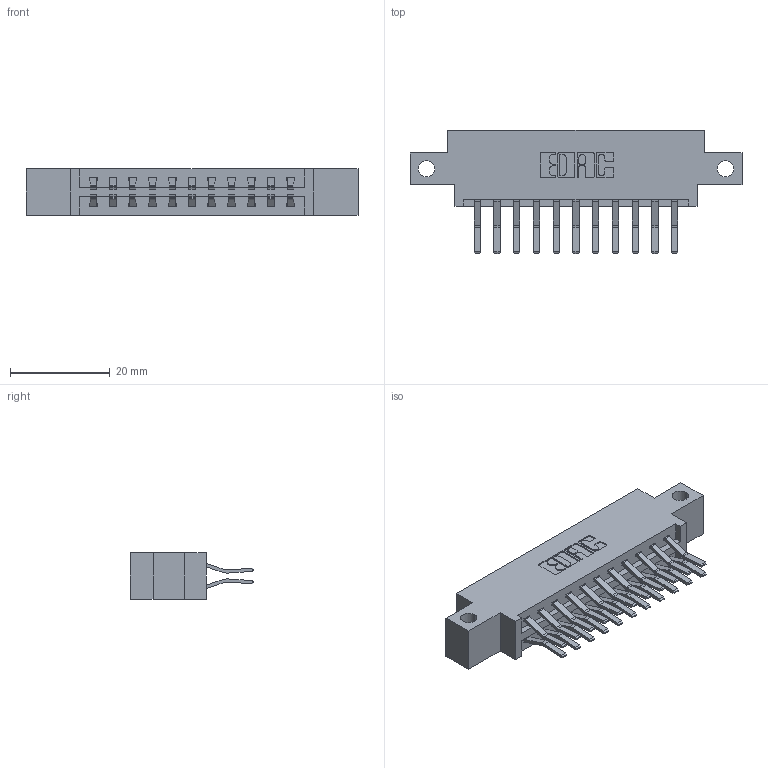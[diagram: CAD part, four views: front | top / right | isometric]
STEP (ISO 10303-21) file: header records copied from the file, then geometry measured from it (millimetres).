
FILE_DESCRIPTION (( 'STEP AP203' ), '1' );
FILE_NAME ('337-022-560-812.STEP', '2018-08-05T16:03:02', ( '' ), ( '' ), 'SwSTEP 2.0', 'SolidWorks 2016', '' );
FILE_SCHEMA (( 'CONFIG_CONTROL_DESIGN' ));
Length unit declared in the file: inch
Products named in the file (3): 337 Part_0.170 Offset - Side Mount; 345-292-001_560 Tail; 337-022-560-812
Assembly tree (23 placements, depth 2):
  337-022-560-812
    337 Part_0.170 Offset - Side Mount
    345-292-001_560 Tail  x22
Bounding box: 66.6 x 24.78 x 9.4 mm (x, y, z)
Volume: 6545.5 mm3; surface area: 7470.5 mm2
Topology: 23 solids, 23 shells, 1350 faces, 3997 edges, 2634 vertices
Faces by surface type: plane 910, cylinder 440
Entity records: 12761 total; most frequent: CARTESIAN_POINT 2178, ORIENTED_EDGE 2114, DIRECTION 1913, EDGE_CURVE 1057, LINE 925, VECTOR 925, VERTEX_POINT 702, AXIS2_PLACEMENT_3D 494
